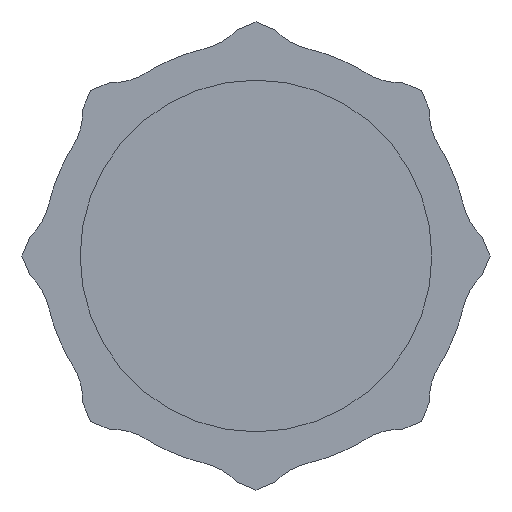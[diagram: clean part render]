
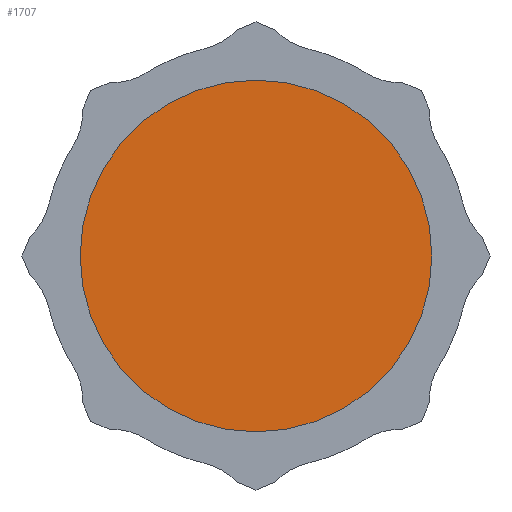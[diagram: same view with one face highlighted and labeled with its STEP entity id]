
A CAD part, front view. The second image highlights one B-rep face of the part: STEP entity #1707.
In plain terms, the highlighted planar face has unit normal (0, -1, 0).
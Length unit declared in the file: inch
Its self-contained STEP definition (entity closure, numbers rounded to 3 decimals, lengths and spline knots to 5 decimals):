
#25=PLANE('',#1934);
#133=CIRCLE('',#1933,0.1305);
#256=FACE_OUTER_BOUND('',#356,.T.);
#356=EDGE_LOOP('',(#1421));
#773=VERTEX_POINT('',#3276);
#1009=EDGE_CURVE('',#773,#773,#133,.T.);
#1421=ORIENTED_EDGE('',*,*,#1009,.T.);
#1707=ADVANCED_FACE('',(#256),#25,.F.);
#1933=AXIS2_PLACEMENT_3D('',#3278,#2413,#2414);
#1934=AXIS2_PLACEMENT_3D('',#3279,#2415,#2416);
#2413=DIRECTION('center_axis',(0.,-1.,0.));
#2414=DIRECTION('ref_axis',(1.,0.,0.));
#2415=DIRECTION('center_axis',(0.,1.,0.));
#2416=DIRECTION('ref_axis',(0.,0.,1.));
#3276=CARTESIAN_POINT('',(-0.1305,1.9,0.));
#3278=CARTESIAN_POINT('Origin',(0.,1.9,0.));
#3279=CARTESIAN_POINT('Origin',(0.,1.9,0.));
